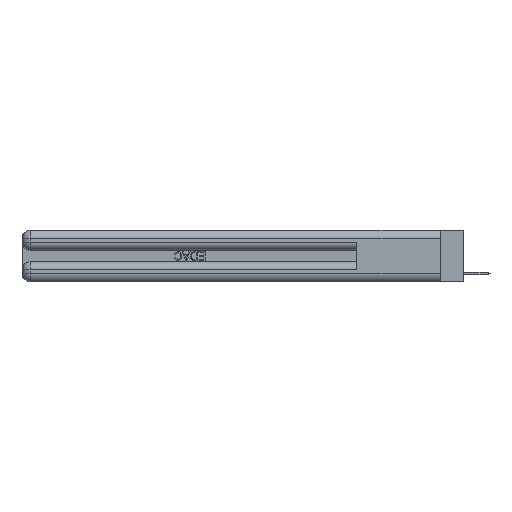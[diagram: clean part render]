
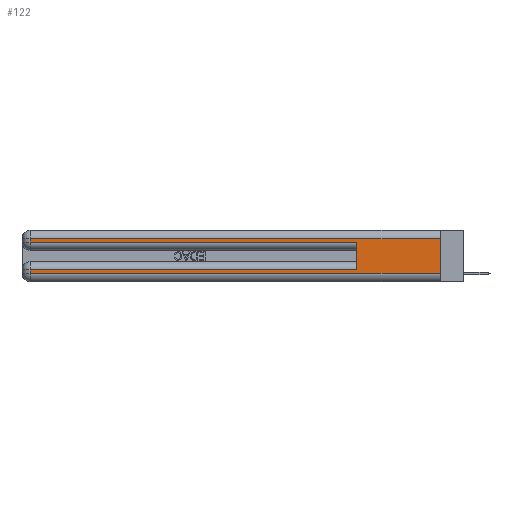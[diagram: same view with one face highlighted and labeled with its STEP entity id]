
A CAD part, left-side view. The second image highlights one B-rep face of the part: STEP entity #122.
In plain terms, the highlighted planar face has unit normal (-1, 0, 0).
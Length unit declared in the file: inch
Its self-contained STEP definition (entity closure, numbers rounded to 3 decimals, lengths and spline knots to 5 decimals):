
#122 = ADVANCED_FACE ( 'NONE', ( #26938 ), #1686, .F. ) ;
#1090 = CARTESIAN_POINT ( 'NONE',  ( 0., 2.94, 0.285 ) ) ;
#1537 = CARTESIAN_POINT ( 'NONE',  ( 0., 0., 0.06 ) ) ;
#1564 = CARTESIAN_POINT ( 'NONE',  ( 0., 0., 0.06 ) ) ;
#1686 = PLANE ( 'NONE',  #29071 ) ;
#2857 = ORIENTED_EDGE ( 'NONE', *, *, #8021, .T. ) ;
#4158 = VERTEX_POINT ( 'NONE', #1090 ) ;
#4608 = VECTOR ( 'NONE', #29212, 39.37008 ) ;
#5012 = CARTESIAN_POINT ( 'NONE',  ( 0., 2.94, 0.37 ) ) ;
#5357 = DIRECTION ( 'NONE',  ( 1., 0., 0. ) ) ;
#6261 = CARTESIAN_POINT ( 'NONE',  ( 0., 0., 0.37 ) ) ;
#6273 = VECTOR ( 'NONE', #9490, 39.37008 ) ;
#6504 = DIRECTION ( 'NONE',  ( 0., 1., 0. ) ) ;
#6711 = CARTESIAN_POINT ( 'NONE',  ( 0., 0., 0.285 ) ) ;
#6749 = VERTEX_POINT ( 'NONE', #17538 ) ;
#7571 = DIRECTION ( 'NONE',  ( 0., 0., -1. ) ) ;
#8021 = EDGE_CURVE ( 'NONE', #6749, #18747, #17524, .T. ) ;
#9226 = ORIENTED_EDGE ( 'NONE', *, *, #29670, .T. ) ;
#9490 = DIRECTION ( 'NONE',  ( 0., -1., 0. ) ) ;
#9980 = LINE ( 'NONE', #25231, #29827 ) ;
#10027 = VERTEX_POINT ( 'NONE', #21955 ) ;
#11193 = EDGE_CURVE ( 'NONE', #6749, #21022, #21410, .T. ) ;
#12277 = LINE ( 'NONE', #5012, #12314 ) ;
#12314 = VECTOR ( 'NONE', #7571, 39.37008 ) ;
#13472 = CARTESIAN_POINT ( 'NONE',  ( 0., 0., 0.37 ) ) ;
#13778 = CARTESIAN_POINT ( 'NONE',  ( 0., 0.6, 0.145 ) ) ;
#14213 = CARTESIAN_POINT ( 'NONE',  ( 0., 2.94, 0.31 ) ) ;
#14601 = EDGE_CURVE ( 'NONE', #17651, #4158, #9980, .T. ) ;
#15189 = ORIENTED_EDGE ( 'NONE', *, *, #24354, .T. ) ;
#15381 = EDGE_LOOP ( 'NONE', ( #23984, #17055, #25924, #15189, #15916, #2857, #27344, #9226 ) ) ;
#15916 = ORIENTED_EDGE ( 'NONE', *, *, #11193, .F. ) ;
#16033 = DIRECTION ( 'NONE',  ( 0., 0., -1. ) ) ;
#16357 = LINE ( 'NONE', #1537, #6273 ) ;
#16869 = CARTESIAN_POINT ( 'NONE',  ( 0., 2.94, 0.085 ) ) ;
#16895 = VECTOR ( 'NONE', #21736, 39.37008 ) ;
#17055 = ORIENTED_EDGE ( 'NONE', *, *, #32013, .T. ) ;
#17524 = LINE ( 'NONE', #25409, #20812 ) ;
#17538 = CARTESIAN_POINT ( 'NONE',  ( 0., 0.6, 0.085 ) ) ;
#17651 = VERTEX_POINT ( 'NONE', #14213 ) ;
#18540 = LINE ( 'NONE', #6711, #29864 ) ;
#18625 = VECTOR ( 'NONE', #6504, 39.37008 ) ;
#18747 = VERTEX_POINT ( 'NONE', #16869 ) ;
#20812 = VECTOR ( 'NONE', #28564, 39.37008 ) ;
#21022 = VERTEX_POINT ( 'NONE', #21520 ) ;
#21410 = LINE ( 'NONE', #13778, #16895 ) ;
#21520 = CARTESIAN_POINT ( 'NONE',  ( 0., 0.6, 0.285 ) ) ;
#21736 = DIRECTION ( 'NONE',  ( 0., 0., 1. ) ) ;
#21955 = CARTESIAN_POINT ( 'NONE',  ( 0., 0., 0.31 ) ) ;
#22746 = DIRECTION ( 'NONE',  ( 0., 0., -1. ) ) ;
#23984 = ORIENTED_EDGE ( 'NONE', *, *, #30704, .F. ) ;
#24343 = LINE ( 'NONE', #27325, #18625 ) ;
#24354 = EDGE_CURVE ( 'NONE', #4158, #21022, #18540, .T. ) ;
#24944 = DIRECTION ( 'NONE',  ( 0., -1., 0. ) ) ;
#25231 = CARTESIAN_POINT ( 'NONE',  ( 0., 2.94, 0.37 ) ) ;
#25409 = CARTESIAN_POINT ( 'NONE',  ( 0., 0., 0.085 ) ) ;
#25924 = ORIENTED_EDGE ( 'NONE', *, *, #14601, .T. ) ;
#26516 = CARTESIAN_POINT ( 'NONE',  ( 0., 2.94, 0.06 ) ) ;
#26762 = VERTEX_POINT ( 'NONE', #1564 ) ;
#26938 = FACE_OUTER_BOUND ( 'NONE', #15381, .T. ) ;
#27068 = EDGE_CURVE ( 'NONE', #18747, #30658, #12277, .T. ) ;
#27325 = CARTESIAN_POINT ( 'NONE',  ( 0., 0., 0.31 ) ) ;
#27344 = ORIENTED_EDGE ( 'NONE', *, *, #27068, .T. ) ;
#28564 = DIRECTION ( 'NONE',  ( 0., 1., 0. ) ) ;
#29071 = AXIS2_PLACEMENT_3D ( 'NONE', #13472, #5357, #16033 ) ;
#29212 = DIRECTION ( 'NONE',  ( 0., 0., -1. ) ) ;
#29670 = EDGE_CURVE ( 'NONE', #30658, #26762, #16357, .T. ) ;
#29827 = VECTOR ( 'NONE', #22746, 39.37008 ) ;
#29864 = VECTOR ( 'NONE', #24944, 39.37008 ) ;
#30658 = VERTEX_POINT ( 'NONE', #26516 ) ;
#30704 = EDGE_CURVE ( 'NONE', #10027, #26762, #32094, .T. ) ;
#32013 = EDGE_CURVE ( 'NONE', #10027, #17651, #24343, .T. ) ;
#32094 = LINE ( 'NONE', #6261, #4608 ) ;
